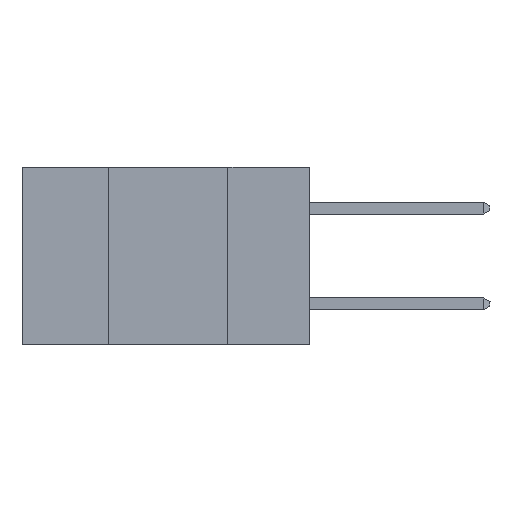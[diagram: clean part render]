
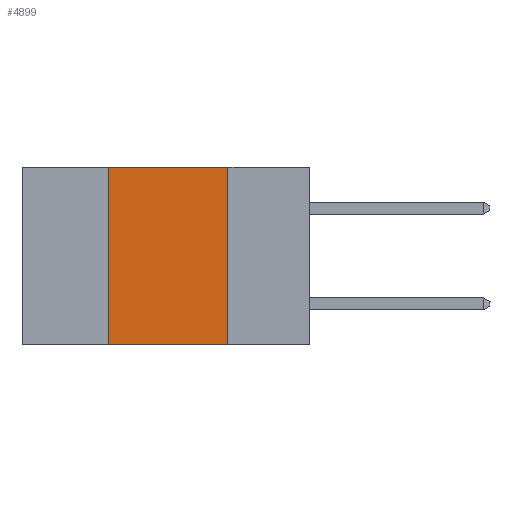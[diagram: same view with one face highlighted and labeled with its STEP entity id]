
A CAD part, left-side view. The second image highlights one B-rep face of the part: STEP entity #4899.
In plain terms, the highlighted planar face has unit normal (-1, 0, 0).
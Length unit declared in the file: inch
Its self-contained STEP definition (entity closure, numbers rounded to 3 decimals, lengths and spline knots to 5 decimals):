
#501 = VERTEX_POINT ( 'NONE', #18261 ) ;
#1211 = ORIENTED_EDGE ( 'NONE', *, *, #25477, .F. ) ;
#1519 = LINE ( 'NONE', #26241, #35431 ) ;
#1880 = CARTESIAN_POINT ( 'NONE',  ( 0., 0.6, 0. ) ) ;
#4875 = LINE ( 'NONE', #25490, #31216 ) ;
#4899 = ADVANCED_FACE ( 'NONE', ( #10925 ), #28760, .F. ) ;
#8068 = ORIENTED_EDGE ( 'NONE', *, *, #24241, .F. ) ;
#9096 = EDGE_LOOP ( 'NONE', ( #27420, #8068, #1211, #36250 ) ) ;
#10870 = CARTESIAN_POINT ( 'NONE',  ( 0., 0.17, -0.37 ) ) ;
#10925 = FACE_OUTER_BOUND ( 'NONE', #9096, .T. ) ;
#14116 = VERTEX_POINT ( 'NONE', #35002 ) ;
#16465 = DIRECTION ( 'NONE',  ( 0., 0., -1. ) ) ;
#16740 = VERTEX_POINT ( 'NONE', #10870 ) ;
#17954 = VECTOR ( 'NONE', #18080, 39.37008 ) ;
#18080 = DIRECTION ( 'NONE',  ( 0., 0., 1. ) ) ;
#18261 = CARTESIAN_POINT ( 'NONE',  ( 0., 0.42, -0.37 ) ) ;
#21426 = CARTESIAN_POINT ( 'NONE',  ( 0., 0.42, 0. ) ) ;
#22192 = VECTOR ( 'NONE', #35374, 39.37008 ) ;
#22899 = DIRECTION ( 'NONE',  ( 0., 0., -1. ) ) ;
#22919 = EDGE_CURVE ( 'NONE', #501, #16740, #35180, .T. ) ;
#23224 = CARTESIAN_POINT ( 'NONE',  ( 0., 0.6, -0.37 ) ) ;
#24241 = EDGE_CURVE ( 'NONE', #14116, #32834, #1519, .T. ) ;
#25477 = EDGE_CURVE ( 'NONE', #501, #14116, #33573, .T. ) ;
#25490 = CARTESIAN_POINT ( 'NONE',  ( 0., 0.17, 0. ) ) ;
#26241 = CARTESIAN_POINT ( 'NONE',  ( 0., 0.6, 0. ) ) ;
#27420 = ORIENTED_EDGE ( 'NONE', *, *, #27441, .F. ) ;
#27441 = EDGE_CURVE ( 'NONE', #32834, #16740, #4875, .T. ) ;
#28760 = PLANE ( 'NONE',  #36412 ) ;
#29179 = DIRECTION ( 'NONE',  ( 0., -1., 0. ) ) ;
#31216 = VECTOR ( 'NONE', #16465, 39.37008 ) ;
#32296 = DIRECTION ( 'NONE',  ( 1., 0., 0. ) ) ;
#32834 = VERTEX_POINT ( 'NONE', #36836 ) ;
#33573 = LINE ( 'NONE', #21426, #17954 ) ;
#35002 = CARTESIAN_POINT ( 'NONE',  ( 0., 0.42, 0. ) ) ;
#35180 = LINE ( 'NONE', #23224, #22192 ) ;
#35374 = DIRECTION ( 'NONE',  ( 0., -1., 0. ) ) ;
#35431 = VECTOR ( 'NONE', #29179, 39.37008 ) ;
#36250 = ORIENTED_EDGE ( 'NONE', *, *, #22919, .T. ) ;
#36412 = AXIS2_PLACEMENT_3D ( 'NONE', #1880, #32296, #22899 ) ;
#36836 = CARTESIAN_POINT ( 'NONE',  ( 0., 0.17, 0. ) ) ;
